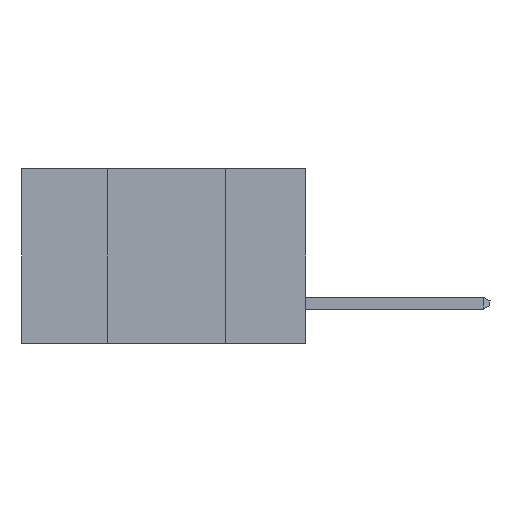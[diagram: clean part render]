
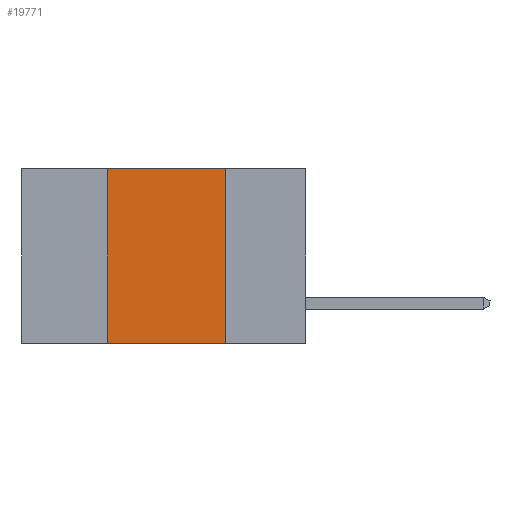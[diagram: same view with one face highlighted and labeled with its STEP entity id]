
A CAD part, left-side view. The second image highlights one B-rep face of the part: STEP entity #19771.
In plain terms, the highlighted planar face has unit normal (-1, 0, 0).
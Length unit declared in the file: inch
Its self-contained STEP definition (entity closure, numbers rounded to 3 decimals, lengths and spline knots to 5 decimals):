
#952 = EDGE_LOOP ( 'NONE', ( #9854, #20110, #15986, #21179 ) ) ;
#1009 = FACE_OUTER_BOUND ( 'NONE', #952, .T. ) ;
#1047 = LINE ( 'NONE', #14604, #1510 ) ;
#1510 = VECTOR ( 'NONE', #7711, 39.37008 ) ;
#2507 = CARTESIAN_POINT ( 'NONE',  ( 0., 0.6, 0. ) ) ;
#3242 = VECTOR ( 'NONE', #7725, 39.37008 ) ;
#3583 = CARTESIAN_POINT ( 'NONE',  ( 0., 0.17, -0.37 ) ) ;
#4705 = EDGE_CURVE ( 'NONE', #11202, #5550, #22420, .T. ) ;
#5550 = VERTEX_POINT ( 'NONE', #12132 ) ;
#6538 = VECTOR ( 'NONE', #15761, 39.37008 ) ;
#6952 = VERTEX_POINT ( 'NONE', #12281 ) ;
#7711 = DIRECTION ( 'NONE',  ( 0., -1., 0. ) ) ;
#7725 = DIRECTION ( 'NONE',  ( 0., -1., 0. ) ) ;
#7758 = CARTESIAN_POINT ( 'NONE',  ( 0., 0.42, -0.37 ) ) ;
#8016 = DIRECTION ( 'NONE',  ( 0., 0., -1. ) ) ;
#8220 = CARTESIAN_POINT ( 'NONE',  ( 0., 0.42, 0. ) ) ;
#8405 = AXIS2_PLACEMENT_3D ( 'NONE', #2507, #15252, #8016 ) ;
#9167 = CARTESIAN_POINT ( 'NONE',  ( 0., 0.17, 0. ) ) ;
#9457 = LINE ( 'NONE', #19792, #3242 ) ;
#9854 = ORIENTED_EDGE ( 'NONE', *, *, #4705, .F. ) ;
#10003 = VERTEX_POINT ( 'NONE', #8220 ) ;
#10119 = EDGE_CURVE ( 'NONE', #6952, #10003, #13393, .T. ) ;
#11202 = VERTEX_POINT ( 'NONE', #9167 ) ;
#12132 = CARTESIAN_POINT ( 'NONE',  ( 0., 0.17, -0.37 ) ) ;
#12281 = CARTESIAN_POINT ( 'NONE',  ( 0., 0.42, -0.37 ) ) ;
#13166 = DIRECTION ( 'NONE',  ( 0., 0., 1. ) ) ;
#13317 = PLANE ( 'NONE',  #8405 ) ;
#13348 = EDGE_CURVE ( 'NONE', #6952, #5550, #9457, .T. ) ;
#13393 = LINE ( 'NONE', #7758, #20274 ) ;
#14604 = CARTESIAN_POINT ( 'NONE',  ( 0., 0.6, 0. ) ) ;
#15252 = DIRECTION ( 'NONE',  ( 1., 0., 0. ) ) ;
#15761 = DIRECTION ( 'NONE',  ( 0., 0., -1. ) ) ;
#15986 = ORIENTED_EDGE ( 'NONE', *, *, #10119, .F. ) ;
#19771 = ADVANCED_FACE ( 'NONE', ( #1009 ), #13317, .F. ) ;
#19792 = CARTESIAN_POINT ( 'NONE',  ( 0., 0.6, -0.37 ) ) ;
#20110 = ORIENTED_EDGE ( 'NONE', *, *, #22516, .F. ) ;
#20274 = VECTOR ( 'NONE', #13166, 39.37008 ) ;
#21179 = ORIENTED_EDGE ( 'NONE', *, *, #13348, .T. ) ;
#22420 = LINE ( 'NONE', #3583, #6538 ) ;
#22516 = EDGE_CURVE ( 'NONE', #10003, #11202, #1047, .T. ) ;
